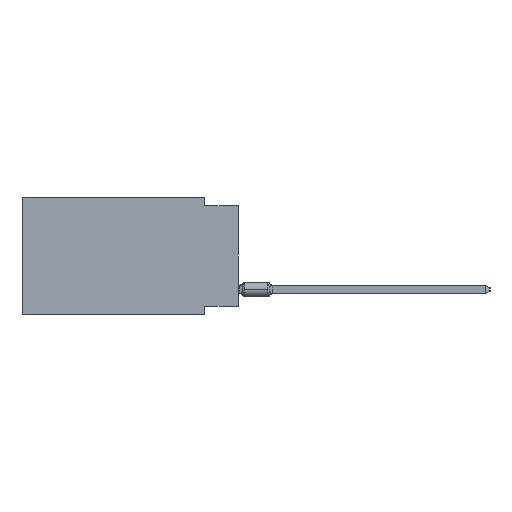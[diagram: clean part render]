
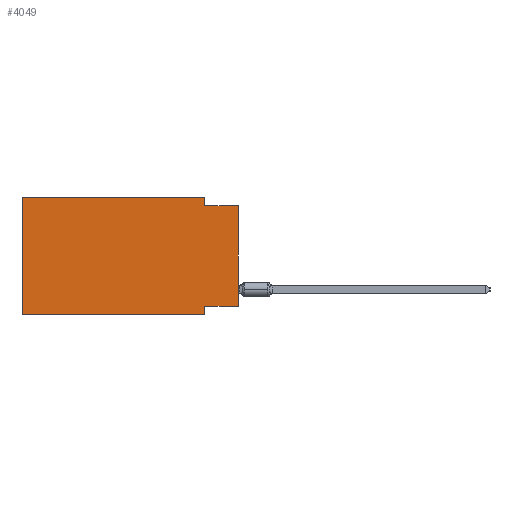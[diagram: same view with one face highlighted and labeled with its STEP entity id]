
A CAD part, left-side view. The second image highlights one B-rep face of the part: STEP entity #4049.
In plain terms, the highlighted planar face has unit normal (-1, 0, 0).
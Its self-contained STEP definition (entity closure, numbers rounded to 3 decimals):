
#1178 = CARTESIAN_POINT ( 'NONE',  ( 0., 16.383, 0. ) ) ;
#3333 = DIRECTION ( 'NONE',  ( 1., 0., 0. ) ) ;
#4049 = ADVANCED_FACE ( 'NONE', ( #26347 ), #21519, .F. ) ;
#4324 = DIRECTION ( 'NONE',  ( 0., 0., 1. ) ) ;
#4342 = EDGE_LOOP ( 'NONE', ( #15620, #50205, #21678, #10982, #14088, #8190, #43682, #23517 ) ) ;
#4931 = CARTESIAN_POINT ( 'NONE',  ( 0., 16.383, 0. ) ) ;
#5378 = CARTESIAN_POINT ( 'NONE',  ( 0., 0., 0. ) ) ;
#5630 = VERTEX_POINT ( 'NONE', #8199 ) ;
#6848 = CARTESIAN_POINT ( 'NONE',  ( 0., 0., -0.635 ) ) ;
#8190 = ORIENTED_EDGE ( 'NONE', *, *, #10789, .T. ) ;
#8197 = EDGE_CURVE ( 'NONE', #57424, #5630, #8627, .T. ) ;
#8199 = CARTESIAN_POINT ( 'NONE',  ( 0., 2.54, -0.635 ) ) ;
#8616 = AXIS2_PLACEMENT_3D ( 'NONE', #44794, #3333, #21802 ) ;
#8627 = LINE ( 'NONE', #27104, #37096 ) ;
#10789 = EDGE_CURVE ( 'NONE', #38650, #59252, #19791, .T. ) ;
#10824 = VECTOR ( 'NONE', #40955, 1000. ) ;
#10845 = LINE ( 'NONE', #1178, #24099 ) ;
#10982 = ORIENTED_EDGE ( 'NONE', *, *, #18616, .F. ) ;
#10989 = DIRECTION ( 'NONE',  ( 0., -1., 0. ) ) ;
#12754 = EDGE_CURVE ( 'NONE', #5630, #18341, #21060, .T. ) ;
#14088 = ORIENTED_EDGE ( 'NONE', *, *, #58725, .F. ) ;
#14511 = CARTESIAN_POINT ( 'NONE',  ( 0., 16.383, 0. ) ) ;
#15272 = VERTEX_POINT ( 'NONE', #14511 ) ;
#15620 = ORIENTED_EDGE ( 'NONE', *, *, #28818, .T. ) ;
#15659 = CARTESIAN_POINT ( 'NONE',  ( 0., 16.383, -8.89 ) ) ;
#18341 = VERTEX_POINT ( 'NONE', #53305 ) ;
#18399 = CARTESIAN_POINT ( 'NONE',  ( 0., 2.54, -8.255 ) ) ;
#18616 = EDGE_CURVE ( 'NONE', #15272, #57424, #10845, .T. ) ;
#19791 = LINE ( 'NONE', #38236, #56587 ) ;
#21060 = LINE ( 'NONE', #6848, #56035 ) ;
#21519 = PLANE ( 'NONE',  #8616 ) ;
#21678 = ORIENTED_EDGE ( 'NONE', *, *, #8197, .F. ) ;
#21802 = DIRECTION ( 'NONE',  ( 0., 0., -1. ) ) ;
#22567 = EDGE_CURVE ( 'NONE', #58527, #57919, #45175, .T. ) ;
#23517 = ORIENTED_EDGE ( 'NONE', *, *, #22567, .F. ) ;
#24099 = VECTOR ( 'NONE', #33263, 1000. ) ;
#26347 = FACE_OUTER_BOUND ( 'NONE', #4342, .T. ) ;
#27104 = CARTESIAN_POINT ( 'NONE',  ( 0., 2.54, 0. ) ) ;
#28818 = EDGE_CURVE ( 'NONE', #58527, #18341, #57128, .T. ) ;
#31896 = VECTOR ( 'NONE', #54315, 1000. ) ;
#33263 = DIRECTION ( 'NONE',  ( 0., -1., 0. ) ) ;
#34992 = DIRECTION ( 'NONE',  ( 0., -1., 0. ) ) ;
#36461 = VECTOR ( 'NONE', #4324, 1000. ) ;
#36487 = VECTOR ( 'NONE', #47449, 1000. ) ;
#37096 = VECTOR ( 'NONE', #55243, 1000. ) ;
#38236 = CARTESIAN_POINT ( 'NONE',  ( 0., 16.383, -8.89 ) ) ;
#38650 = VERTEX_POINT ( 'NONE', #15659 ) ;
#39163 = CARTESIAN_POINT ( 'NONE',  ( 0., 2.54, -8.89 ) ) ;
#40953 = LINE ( 'NONE', #4931, #36461 ) ;
#40955 = DIRECTION ( 'NONE',  ( 0., 1., 0. ) ) ;
#41743 = EDGE_CURVE ( 'NONE', #57919, #59252, #53416, .T. ) ;
#42071 = CARTESIAN_POINT ( 'NONE',  ( 0., 2.54, -8.89 ) ) ;
#43682 = ORIENTED_EDGE ( 'NONE', *, *, #41743, .F. ) ;
#43689 = CARTESIAN_POINT ( 'NONE',  ( 0., 2.54, 0. ) ) ;
#44794 = CARTESIAN_POINT ( 'NONE',  ( 0., 16.383, 0. ) ) ;
#45175 = LINE ( 'NONE', #45498, #10824 ) ;
#45498 = CARTESIAN_POINT ( 'NONE',  ( 0., 0., -8.255 ) ) ;
#47449 = DIRECTION ( 'NONE',  ( 0., 0., 1. ) ) ;
#50205 = ORIENTED_EDGE ( 'NONE', *, *, #12754, .F. ) ;
#53305 = CARTESIAN_POINT ( 'NONE',  ( 0., 0., -0.635 ) ) ;
#53392 = CARTESIAN_POINT ( 'NONE',  ( 0., 0., -8.255 ) ) ;
#53416 = LINE ( 'NONE', #39163, #31896 ) ;
#54315 = DIRECTION ( 'NONE',  ( 0., 0., -1. ) ) ;
#55243 = DIRECTION ( 'NONE',  ( 0., 0., -1. ) ) ;
#56035 = VECTOR ( 'NONE', #34992, 1000. ) ;
#56587 = VECTOR ( 'NONE', #10989, 1000. ) ;
#57128 = LINE ( 'NONE', #5378, #36487 ) ;
#57424 = VERTEX_POINT ( 'NONE', #43689 ) ;
#57919 = VERTEX_POINT ( 'NONE', #18399 ) ;
#58527 = VERTEX_POINT ( 'NONE', #53392 ) ;
#58725 = EDGE_CURVE ( 'NONE', #38650, #15272, #40953, .T. ) ;
#59252 = VERTEX_POINT ( 'NONE', #42071 ) ;
